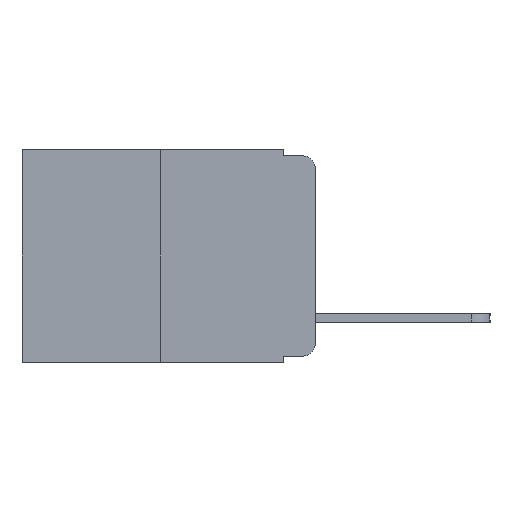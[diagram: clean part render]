
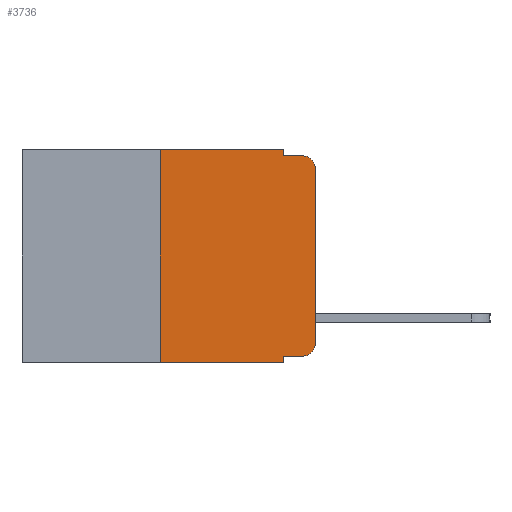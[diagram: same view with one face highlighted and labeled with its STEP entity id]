
A CAD part, left-side view. The second image highlights one B-rep face of the part: STEP entity #3736.
In plain terms, the highlighted planar face has unit normal (-1, 0, 0).
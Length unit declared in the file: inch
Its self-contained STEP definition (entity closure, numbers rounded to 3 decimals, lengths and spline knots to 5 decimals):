
#17 = ORIENTED_EDGE ( 'NONE', *, *, #7313, .F. ) ;
#647 = CARTESIAN_POINT ( 'NONE',  ( 0., 0.02, -0.333 ) ) ;
#1329 = ORIENTED_EDGE ( 'NONE', *, *, #6173, .T. ) ;
#2030 = CARTESIAN_POINT ( 'NONE',  ( 0., 0.051, -0.01 ) ) ;
#2363 = EDGE_CURVE ( 'NONE', #14465, #15869, #13841, .T. ) ;
#2365 = CARTESIAN_POINT ( 'NONE',  ( 0., 0.051, -0.343 ) ) ;
#2584 = CARTESIAN_POINT ( 'NONE',  ( 0., 0.051, -0.01 ) ) ;
#2585 = VECTOR ( 'NONE', #3827, 39.37008 ) ;
#2673 = DIRECTION ( 'NONE',  ( 0., 0., -1. ) ) ;
#2952 = ORIENTED_EDGE ( 'NONE', *, *, #11334, .F. ) ;
#3022 = DIRECTION ( 'NONE',  ( -1., 0., 0. ) ) ;
#3295 = DIRECTION ( 'NONE',  ( 0., -1., 0. ) ) ;
#3335 = LINE ( 'NONE', #19127, #18543 ) ;
#3736 = ADVANCED_FACE ( 'NONE', ( #5472 ), #12374, .F. ) ;
#3827 = DIRECTION ( 'NONE',  ( 0., 0., 1. ) ) ;
#4074 = VERTEX_POINT ( 'NONE', #2365 ) ;
#4479 = DIRECTION ( 'NONE',  ( 0., 0., -1. ) ) ;
#5398 = VERTEX_POINT ( 'NONE', #7133 ) ;
#5403 = CARTESIAN_POINT ( 'NONE',  ( 0., 0.25, 0. ) ) ;
#5472 = FACE_OUTER_BOUND ( 'NONE', #6189, .T. ) ;
#5999 = VECTOR ( 'NONE', #19093, 39.37008 ) ;
#6173 = EDGE_CURVE ( 'NONE', #8750, #4074, #3335, .T. ) ;
#6189 = EDGE_LOOP ( 'NONE', ( #7464, #12843, #18212, #2952, #9354, #7561, #1329, #17, #6550, #17446 ) ) ;
#6256 = VECTOR ( 'NONE', #7774, 39.37008 ) ;
#6293 = EDGE_CURVE ( 'NONE', #10099, #14465, #8901, .T. ) ;
#6481 = CARTESIAN_POINT ( 'NONE',  ( 0., 0.051, 0. ) ) ;
#6507 = CARTESIAN_POINT ( 'NONE',  ( 0., 0., -0.313 ) ) ;
#6550 = ORIENTED_EDGE ( 'NONE', *, *, #6293, .T. ) ;
#6904 = VECTOR ( 'NONE', #13895, 39.37008 ) ;
#7133 = CARTESIAN_POINT ( 'NONE',  ( 0., 0., -0.03 ) ) ;
#7306 = AXIS2_PLACEMENT_3D ( 'NONE', #11927, #3022, #13383 ) ;
#7313 = EDGE_CURVE ( 'NONE', #10099, #4074, #17811, .T. ) ;
#7320 = CARTESIAN_POINT ( 'NONE',  ( 0., 0.051, 0. ) ) ;
#7464 = ORIENTED_EDGE ( 'NONE', *, *, #17202, .T. ) ;
#7561 = ORIENTED_EDGE ( 'NONE', *, *, #8320, .F. ) ;
#7686 = CARTESIAN_POINT ( 'NONE',  ( 0., 0.473, 0. ) ) ;
#7707 = CARTESIAN_POINT ( 'NONE',  ( 0., 0.473, 0. ) ) ;
#7756 = VERTEX_POINT ( 'NONE', #5403 ) ;
#7774 = DIRECTION ( 'NONE',  ( 0., -1., 0. ) ) ;
#8096 = LINE ( 'NONE', #12814, #16409 ) ;
#8320 = EDGE_CURVE ( 'NONE', #8750, #7756, #8096, .T. ) ;
#8750 = VERTEX_POINT ( 'NONE', #9366 ) ;
#8884 = DIRECTION ( 'NONE',  ( 0., -1., 0. ) ) ;
#8901 = LINE ( 'NONE', #12193, #16268 ) ;
#9354 = ORIENTED_EDGE ( 'NONE', *, *, #16993, .F. ) ;
#9366 = CARTESIAN_POINT ( 'NONE',  ( 0., 0.25, -0.343 ) ) ;
#10099 = VERTEX_POINT ( 'NONE', #12525 ) ;
#10349 = CARTESIAN_POINT ( 'NONE',  ( 0., 0.02, -0.313 ) ) ;
#10501 = LINE ( 'NONE', #17051, #2585 ) ;
#10932 = LINE ( 'NONE', #2030, #6904 ) ;
#11334 = EDGE_CURVE ( 'NONE', #16485, #16080, #16217, .T. ) ;
#11579 = CARTESIAN_POINT ( 'NONE',  ( 0., 0.051, 0. ) ) ;
#11927 = CARTESIAN_POINT ( 'NONE',  ( 0., 0.02, -0.03 ) ) ;
#12193 = CARTESIAN_POINT ( 'NONE',  ( 0., 0.051, -0.333 ) ) ;
#12320 = EDGE_CURVE ( 'NONE', #16080, #18150, #10932, .T. ) ;
#12374 = PLANE ( 'NONE',  #18264 ) ;
#12525 = CARTESIAN_POINT ( 'NONE',  ( 0., 0.051, -0.333 ) ) ;
#12786 = VECTOR ( 'NONE', #2673, 39.37008 ) ;
#12814 = CARTESIAN_POINT ( 'NONE',  ( 0., 0.25, 0. ) ) ;
#12843 = ORIENTED_EDGE ( 'NONE', *, *, #16245, .T. ) ;
#13210 = AXIS2_PLACEMENT_3D ( 'NONE', #10349, #18138, #17776 ) ;
#13281 = CIRCLE ( 'NONE', #7306, 0.02 ) ;
#13383 = DIRECTION ( 'NONE',  ( 0., 0., -1. ) ) ;
#13841 = CIRCLE ( 'NONE', #13210, 0.02 ) ;
#13895 = DIRECTION ( 'NONE',  ( 0., -1., 0. ) ) ;
#14275 = DIRECTION ( 'NONE',  ( 0., 0., 1. ) ) ;
#14465 = VERTEX_POINT ( 'NONE', #647 ) ;
#15618 = DIRECTION ( 'NONE',  ( 1., 0., 0. ) ) ;
#15869 = VERTEX_POINT ( 'NONE', #6507 ) ;
#16080 = VERTEX_POINT ( 'NONE', #2584 ) ;
#16217 = LINE ( 'NONE', #11579, #12786 ) ;
#16245 = EDGE_CURVE ( 'NONE', #5398, #18150, #13281, .T. ) ;
#16268 = VECTOR ( 'NONE', #3295, 39.37008 ) ;
#16409 = VECTOR ( 'NONE', #14275, 39.37008 ) ;
#16443 = CARTESIAN_POINT ( 'NONE',  ( 0., 0.02, -0.01 ) ) ;
#16485 = VERTEX_POINT ( 'NONE', #6481 ) ;
#16993 = EDGE_CURVE ( 'NONE', #7756, #16485, #18074, .T. ) ;
#17051 = CARTESIAN_POINT ( 'NONE',  ( 0., 0., 0. ) ) ;
#17202 = EDGE_CURVE ( 'NONE', #15869, #5398, #10501, .T. ) ;
#17446 = ORIENTED_EDGE ( 'NONE', *, *, #2363, .T. ) ;
#17776 = DIRECTION ( 'NONE',  ( 0., 0., -1. ) ) ;
#17811 = LINE ( 'NONE', #7320, #5999 ) ;
#18074 = LINE ( 'NONE', #7707, #6256 ) ;
#18138 = DIRECTION ( 'NONE',  ( -1., 0., 0. ) ) ;
#18150 = VERTEX_POINT ( 'NONE', #16443 ) ;
#18212 = ORIENTED_EDGE ( 'NONE', *, *, #12320, .F. ) ;
#18264 = AXIS2_PLACEMENT_3D ( 'NONE', #7686, #15618, #4479 ) ;
#18543 = VECTOR ( 'NONE', #8884, 39.37008 ) ;
#19093 = DIRECTION ( 'NONE',  ( 0., 0., -1. ) ) ;
#19127 = CARTESIAN_POINT ( 'NONE',  ( 0., 0.473, -0.343 ) ) ;
